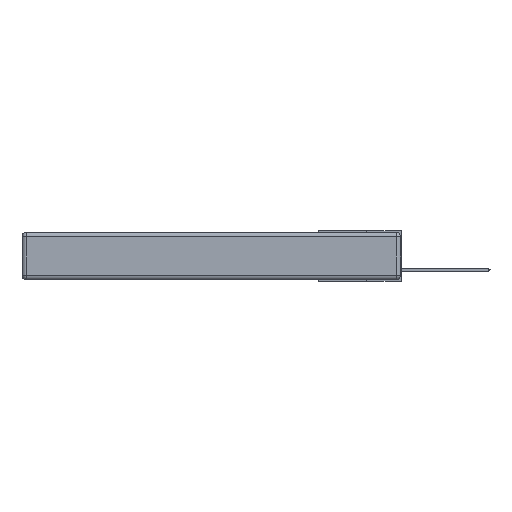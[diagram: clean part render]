
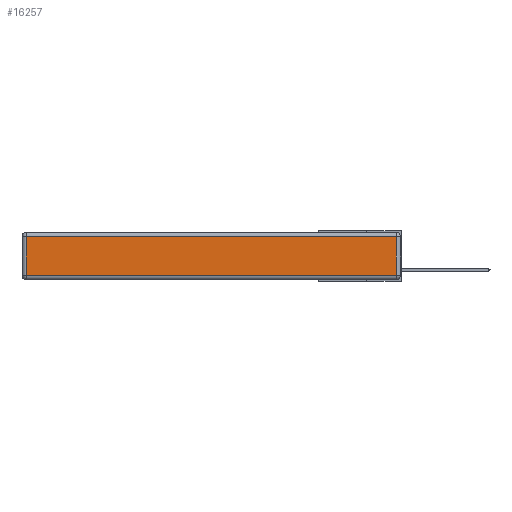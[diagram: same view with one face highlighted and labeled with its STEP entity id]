
A CAD part, left-side view. The second image highlights one B-rep face of the part: STEP entity #16257.
In plain terms, the highlighted planar face has unit normal (-1, 0, 0).
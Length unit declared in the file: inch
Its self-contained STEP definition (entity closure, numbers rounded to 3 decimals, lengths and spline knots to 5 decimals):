
#686 = EDGE_LOOP ( 'NONE', ( #2511, #15997, #7266, #9158 ) ) ;
#1650 = VECTOR ( 'NONE', #3247, 39.37008 ) ;
#2263 = VECTOR ( 'NONE', #3485, 39.37008 ) ;
#2306 = CARTESIAN_POINT ( 'NONE',  ( 0., 2.75, -0.03 ) ) ;
#2511 = ORIENTED_EDGE ( 'NONE', *, *, #18009, .T. ) ;
#3114 = VERTEX_POINT ( 'NONE', #7428 ) ;
#3158 = FACE_OUTER_BOUND ( 'NONE', #686, .T. ) ;
#3247 = DIRECTION ( 'NONE',  ( 0., 0., 1. ) ) ;
#3485 = DIRECTION ( 'NONE',  ( 0., 0., -1. ) ) ;
#4110 = VERTEX_POINT ( 'NONE', #11596 ) ;
#4433 = CARTESIAN_POINT ( 'NONE',  ( 0., 0., -0.343 ) ) ;
#4985 = VERTEX_POINT ( 'NONE', #18207 ) ;
#5436 = VERTEX_POINT ( 'NONE', #9854 ) ;
#6408 = VECTOR ( 'NONE', #17879, 39.37008 ) ;
#7266 = ORIENTED_EDGE ( 'NONE', *, *, #17861, .T. ) ;
#7428 = CARTESIAN_POINT ( 'NONE',  ( 0., 0.03, -0.313 ) ) ;
#7475 = EDGE_CURVE ( 'NONE', #3114, #4985, #17904, .T. ) ;
#7774 = CARTESIAN_POINT ( 'NONE',  ( 0., 0., -0.313 ) ) ;
#9158 = ORIENTED_EDGE ( 'NONE', *, *, #9246, .T. ) ;
#9246 = EDGE_CURVE ( 'NONE', #4110, #5436, #13967, .T. ) ;
#9794 = CARTESIAN_POINT ( 'NONE',  ( 0., 0.03, -0.343 ) ) ;
#9854 = CARTESIAN_POINT ( 'NONE',  ( 0., 2.72, -0.313 ) ) ;
#11113 = LINE ( 'NONE', #2306, #12691 ) ;
#11596 = CARTESIAN_POINT ( 'NONE',  ( 0., 2.72, -0.03 ) ) ;
#12013 = CARTESIAN_POINT ( 'NONE',  ( 0., 2.72, -0.343 ) ) ;
#12447 = LINE ( 'NONE', #7774, #6408 ) ;
#12691 = VECTOR ( 'NONE', #13878, 39.37008 ) ;
#13037 = PLANE ( 'NONE',  #16908 ) ;
#13878 = DIRECTION ( 'NONE',  ( 0., 1., 0. ) ) ;
#13967 = LINE ( 'NONE', #12013, #2263 ) ;
#14508 = DIRECTION ( 'NONE',  ( -1., 0., 0. ) ) ;
#15954 = DIRECTION ( 'NONE',  ( 0., 0., 1. ) ) ;
#15997 = ORIENTED_EDGE ( 'NONE', *, *, #7475, .T. ) ;
#16257 = ADVANCED_FACE ( 'NONE', ( #3158 ), #13037, .T. ) ;
#16908 = AXIS2_PLACEMENT_3D ( 'NONE', #4433, #14508, #15954 ) ;
#17861 = EDGE_CURVE ( 'NONE', #4985, #4110, #11113, .T. ) ;
#17879 = DIRECTION ( 'NONE',  ( 0., -1., 0. ) ) ;
#17904 = LINE ( 'NONE', #9794, #1650 ) ;
#18009 = EDGE_CURVE ( 'NONE', #5436, #3114, #12447, .T. ) ;
#18207 = CARTESIAN_POINT ( 'NONE',  ( 0., 0.03, -0.03 ) ) ;
